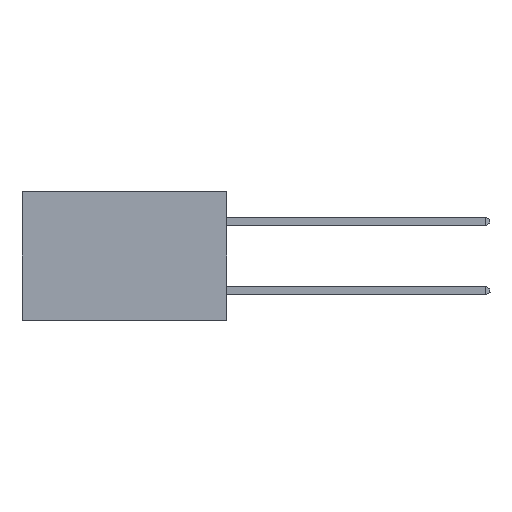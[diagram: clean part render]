
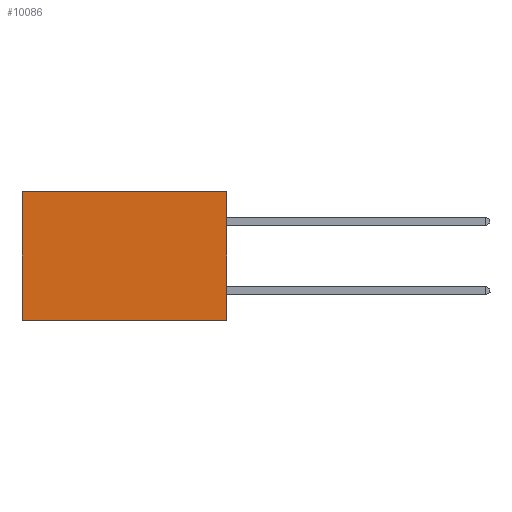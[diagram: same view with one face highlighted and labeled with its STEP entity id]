
A CAD part, left-side view. The second image highlights one B-rep face of the part: STEP entity #10086.
In plain terms, the highlighted planar face has unit normal (-1, 0, 0).
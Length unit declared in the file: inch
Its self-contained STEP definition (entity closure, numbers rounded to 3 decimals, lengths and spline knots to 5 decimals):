
#229 = AXIS2_PLACEMENT_3D ( 'NONE', #8853, #4369, #14670 ) ;
#880 = VECTOR ( 'NONE', #7881, 39.37008 ) ;
#1793 = DIRECTION ( 'NONE',  ( 0., 1., 0. ) ) ;
#3622 = CARTESIAN_POINT ( 'NONE',  ( 0.277, 0., 0. ) ) ;
#3976 = CARTESIAN_POINT ( 'NONE',  ( 0.277, 0.59, 0. ) ) ;
#4162 = EDGE_LOOP ( 'NONE', ( #18927, #10023, #9875, #15528 ) ) ;
#4369 = DIRECTION ( 'NONE',  ( 1., 0., 0. ) ) ;
#4910 = CARTESIAN_POINT ( 'NONE',  ( 0.277, 0.59, -0.37 ) ) ;
#5819 = DIRECTION ( 'NONE',  ( 0., 0., -1. ) ) ;
#7341 = LINE ( 'NONE', #13610, #18432 ) ;
#7881 = DIRECTION ( 'NONE',  ( 0., 0., -1. ) ) ;
#8093 = FACE_OUTER_BOUND ( 'NONE', #4162, .T. ) ;
#8853 = CARTESIAN_POINT ( 'NONE',  ( 0.277, 0., -0.37 ) ) ;
#9361 = VERTEX_POINT ( 'NONE', #11663 ) ;
#9875 = ORIENTED_EDGE ( 'NONE', *, *, #18128, .F. ) ;
#10023 = ORIENTED_EDGE ( 'NONE', *, *, #13810, .F. ) ;
#10086 = ADVANCED_FACE ( 'NONE', ( #8093 ), #13251, .F. ) ;
#10475 = VERTEX_POINT ( 'NONE', #3976 ) ;
#11663 = CARTESIAN_POINT ( 'NONE',  ( 0.277, 0.59, -0.37 ) ) ;
#11857 = VERTEX_POINT ( 'NONE', #18463 ) ;
#12450 = DIRECTION ( 'NONE',  ( 0., 1., 0. ) ) ;
#12749 = LINE ( 'NONE', #14612, #16094 ) ;
#13210 = LINE ( 'NONE', #4910, #880 ) ;
#13251 = PLANE ( 'NONE',  #229 ) ;
#13405 = VECTOR ( 'NONE', #12450, 39.37008 ) ;
#13610 = CARTESIAN_POINT ( 'NONE',  ( 0.277, 0., -0.37 ) ) ;
#13756 = CARTESIAN_POINT ( 'NONE',  ( 0.277, 0., 0. ) ) ;
#13810 = EDGE_CURVE ( 'NONE', #11857, #9361, #7341, .T. ) ;
#14612 = CARTESIAN_POINT ( 'NONE',  ( 0.277, 0., -0.37 ) ) ;
#14670 = DIRECTION ( 'NONE',  ( 0., 0., -1. ) ) ;
#15216 = VERTEX_POINT ( 'NONE', #3622 ) ;
#15528 = ORIENTED_EDGE ( 'NONE', *, *, #18311, .T. ) ;
#16094 = VECTOR ( 'NONE', #5819, 39.37008 ) ;
#17638 = LINE ( 'NONE', #13756, #13405 ) ;
#17708 = EDGE_CURVE ( 'NONE', #10475, #9361, #13210, .T. ) ;
#18128 = EDGE_CURVE ( 'NONE', #15216, #11857, #12749, .T. ) ;
#18311 = EDGE_CURVE ( 'NONE', #15216, #10475, #17638, .T. ) ;
#18432 = VECTOR ( 'NONE', #1793, 39.37008 ) ;
#18463 = CARTESIAN_POINT ( 'NONE',  ( 0.277, 0., -0.37 ) ) ;
#18927 = ORIENTED_EDGE ( 'NONE', *, *, #17708, .T. ) ;
